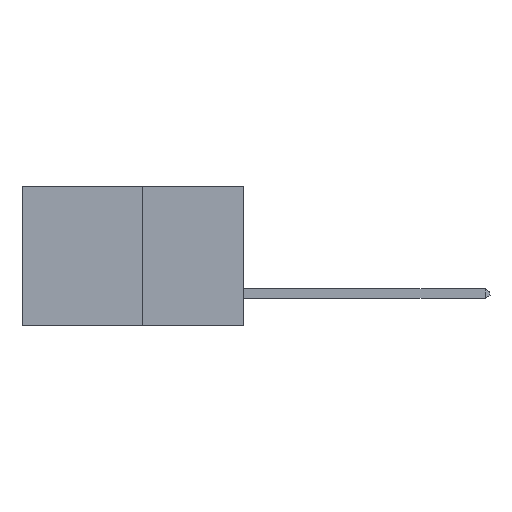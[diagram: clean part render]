
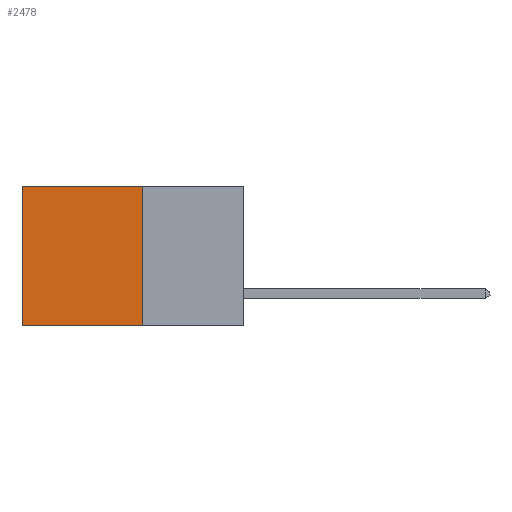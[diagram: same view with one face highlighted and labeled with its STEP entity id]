
A CAD part, left-side view. The second image highlights one B-rep face of the part: STEP entity #2478.
In plain terms, the highlighted planar face has unit normal (-1, 0, 0).
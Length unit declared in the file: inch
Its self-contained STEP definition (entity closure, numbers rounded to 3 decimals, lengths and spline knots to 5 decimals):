
#209 = AXIS2_PLACEMENT_3D ( 'NONE', #8904, #8439, #8209 ) ;
#295 = VECTOR ( 'NONE', #8949, 39.37008 ) ;
#910 = CARTESIAN_POINT ( 'NONE',  ( 0.277, 0.27, 0. ) ) ;
#1008 = DIRECTION ( 'NONE',  ( 0., 1., 0. ) ) ;
#1110 = VERTEX_POINT ( 'NONE', #4375 ) ;
#1324 = LINE ( 'NONE', #910, #3745 ) ;
#2363 = ORIENTED_EDGE ( 'NONE', *, *, #8810, .F. ) ;
#2478 = ADVANCED_FACE ( 'NONE', ( #7213 ), #10623, .F. ) ;
#2829 = CARTESIAN_POINT ( 'NONE',  ( 0.277, 0.27, 0. ) ) ;
#2891 = CARTESIAN_POINT ( 'NONE',  ( 0.277, 0.27, -0.37 ) ) ;
#3298 = VERTEX_POINT ( 'NONE', #11229 ) ;
#3500 = EDGE_CURVE ( 'NONE', #3298, #6836, #7619, .T. ) ;
#3745 = VECTOR ( 'NONE', #1008, 39.37008 ) ;
#3888 = DIRECTION ( 'NONE',  ( 0., 0., -1. ) ) ;
#3958 = LINE ( 'NONE', #2891, #10981 ) ;
#4338 = EDGE_CURVE ( 'NONE', #5102, #3298, #1324, .T. ) ;
#4375 = CARTESIAN_POINT ( 'NONE',  ( 0.277, 0.27, -0.37 ) ) ;
#5102 = VERTEX_POINT ( 'NONE', #2829 ) ;
#5443 = EDGE_CURVE ( 'NONE', #1110, #6836, #7879, .T. ) ;
#6836 = VERTEX_POINT ( 'NONE', #11844 ) ;
#6894 = CARTESIAN_POINT ( 'NONE',  ( 0.277, 0.59, -0.37 ) ) ;
#6901 = DIRECTION ( 'NONE',  ( 0., 0., -1. ) ) ;
#6953 = ORIENTED_EDGE ( 'NONE', *, *, #5443, .F. ) ;
#7213 = FACE_OUTER_BOUND ( 'NONE', #11413, .T. ) ;
#7233 = ORIENTED_EDGE ( 'NONE', *, *, #4338, .T. ) ;
#7619 = LINE ( 'NONE', #6894, #9714 ) ;
#7879 = LINE ( 'NONE', #8888, #295 ) ;
#8209 = DIRECTION ( 'NONE',  ( 0., 0., -1. ) ) ;
#8439 = DIRECTION ( 'NONE',  ( 1., 0., 0. ) ) ;
#8810 = EDGE_CURVE ( 'NONE', #5102, #1110, #3958, .T. ) ;
#8888 = CARTESIAN_POINT ( 'NONE',  ( 0.277, 0.27, -0.37 ) ) ;
#8904 = CARTESIAN_POINT ( 'NONE',  ( 0.277, 0.27, -0.37 ) ) ;
#8949 = DIRECTION ( 'NONE',  ( 0., 1., 0. ) ) ;
#9714 = VECTOR ( 'NONE', #6901, 39.37008 ) ;
#10623 = PLANE ( 'NONE',  #209 ) ;
#10981 = VECTOR ( 'NONE', #3888, 39.37008 ) ;
#11229 = CARTESIAN_POINT ( 'NONE',  ( 0.277, 0.59, 0. ) ) ;
#11351 = ORIENTED_EDGE ( 'NONE', *, *, #3500, .T. ) ;
#11413 = EDGE_LOOP ( 'NONE', ( #11351, #6953, #2363, #7233 ) ) ;
#11844 = CARTESIAN_POINT ( 'NONE',  ( 0.277, 0.59, -0.37 ) ) ;
